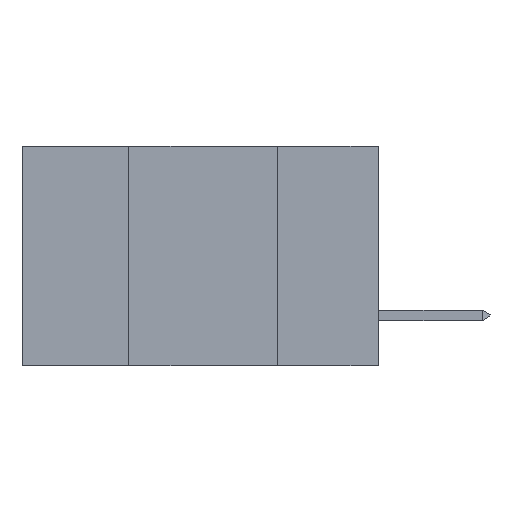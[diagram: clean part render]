
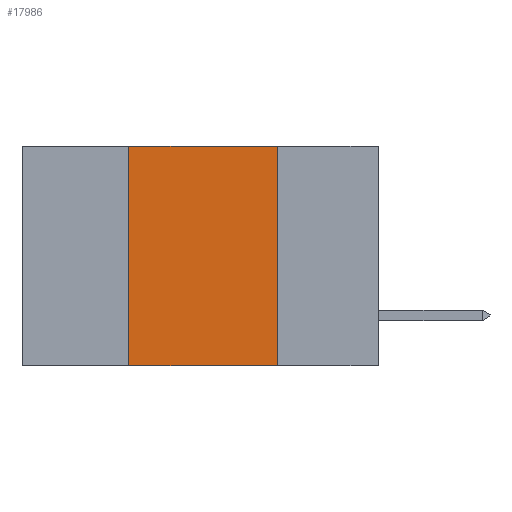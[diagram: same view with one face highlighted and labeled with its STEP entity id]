
A CAD part, left-side view. The second image highlights one B-rep face of the part: STEP entity #17986.
In plain terms, the highlighted planar face has unit normal (-1, 0, 0).
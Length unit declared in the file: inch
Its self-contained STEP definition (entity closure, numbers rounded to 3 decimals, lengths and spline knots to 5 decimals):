
#1661 = VERTEX_POINT ( 'NONE', #15196 ) ;
#2070 = LINE ( 'NONE', #18650, #17579 ) ;
#2081 = ORIENTED_EDGE ( 'NONE', *, *, #7625, .T. ) ;
#3406 = CARTESIAN_POINT ( 'NONE',  ( 0., 0.42, 0. ) ) ;
#3627 = LINE ( 'NONE', #15493, #3950 ) ;
#3749 = DIRECTION ( 'NONE',  ( 0., 0., -1. ) ) ;
#3913 = DIRECTION ( 'NONE',  ( 0., 0., -1. ) ) ;
#3950 = VECTOR ( 'NONE', #3913, 39.37008 ) ;
#5072 = DIRECTION ( 'NONE',  ( 0., -1., 0. ) ) ;
#5492 = PLANE ( 'NONE',  #12247 ) ;
#6801 = CARTESIAN_POINT ( 'NONE',  ( 0., 0.6, -0.37 ) ) ;
#6995 = EDGE_CURVE ( 'NONE', #12330, #19002, #2070, .T. ) ;
#7126 = FACE_OUTER_BOUND ( 'NONE', #19071, .T. ) ;
#7625 = EDGE_CURVE ( 'NONE', #1661, #8334, #15662, .T. ) ;
#7809 = LINE ( 'NONE', #16394, #15612 ) ;
#8334 = VERTEX_POINT ( 'NONE', #11657 ) ;
#9050 = EDGE_CURVE ( 'NONE', #19002, #8334, #3627, .T. ) ;
#9952 = CARTESIAN_POINT ( 'NONE',  ( 0., 0.6, 0. ) ) ;
#11421 = DIRECTION ( 'NONE',  ( 1., 0., 0. ) ) ;
#11657 = CARTESIAN_POINT ( 'NONE',  ( 0., 0.17, -0.37 ) ) ;
#12157 = ORIENTED_EDGE ( 'NONE', *, *, #14442, .F. ) ;
#12247 = AXIS2_PLACEMENT_3D ( 'NONE', #9952, #11421, #3749 ) ;
#12330 = VERTEX_POINT ( 'NONE', #3406 ) ;
#13896 = VECTOR ( 'NONE', #18560, 39.37008 ) ;
#14146 = CARTESIAN_POINT ( 'NONE',  ( 0., 0.17, 0. ) ) ;
#14442 = EDGE_CURVE ( 'NONE', #1661, #12330, #7809, .T. ) ;
#14962 = ORIENTED_EDGE ( 'NONE', *, *, #9050, .F. ) ;
#15140 = DIRECTION ( 'NONE',  ( 0., 0., 1. ) ) ;
#15196 = CARTESIAN_POINT ( 'NONE',  ( 0., 0.42, -0.37 ) ) ;
#15493 = CARTESIAN_POINT ( 'NONE',  ( 0., 0.17, -0.37 ) ) ;
#15612 = VECTOR ( 'NONE', #15140, 39.37008 ) ;
#15662 = LINE ( 'NONE', #6801, #13896 ) ;
#16394 = CARTESIAN_POINT ( 'NONE',  ( 0., 0.42, -0.37 ) ) ;
#16464 = ORIENTED_EDGE ( 'NONE', *, *, #6995, .F. ) ;
#17579 = VECTOR ( 'NONE', #5072, 39.37008 ) ;
#17986 = ADVANCED_FACE ( 'NONE', ( #7126 ), #5492, .F. ) ;
#18560 = DIRECTION ( 'NONE',  ( 0., -1., 0. ) ) ;
#18650 = CARTESIAN_POINT ( 'NONE',  ( 0., 0.6, 0. ) ) ;
#19002 = VERTEX_POINT ( 'NONE', #14146 ) ;
#19071 = EDGE_LOOP ( 'NONE', ( #14962, #16464, #12157, #2081 ) ) ;
